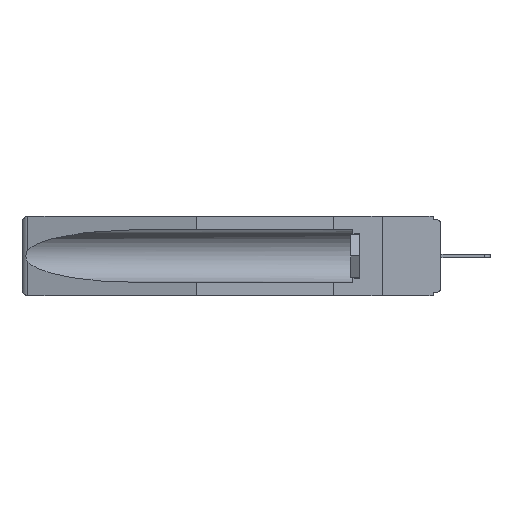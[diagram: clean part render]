
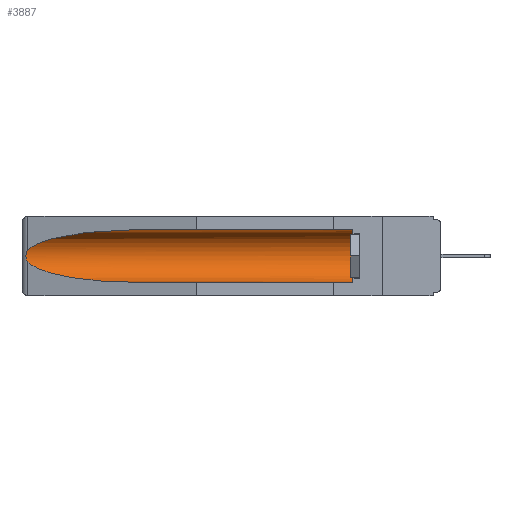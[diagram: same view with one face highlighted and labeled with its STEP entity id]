
A CAD part, left-side view. The second image highlights one B-rep face of the part: STEP entity #3887.
In plain terms, the highlighted cylindrical face has radius 2.857 mm (diameter 5.715 mm), a partial arc.
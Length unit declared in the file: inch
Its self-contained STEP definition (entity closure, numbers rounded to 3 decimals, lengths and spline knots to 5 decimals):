
#314 = ORIENTED_EDGE ( 'NONE', *, *, #5196, .T. ) ;
#578 = ORIENTED_EDGE ( 'NONE', *, *, #16388, .T. ) ;
#771 = LINE ( 'NONE', #19062, #4233 ) ;
#824 = DIRECTION ( 'NONE',  ( 0., 1., 0. ) ) ;
#1317 = CARTESIAN_POINT ( 'NONE',  ( 0.155, 0.126, -0.059 ) ) ;
#1935 = ORIENTED_EDGE ( 'NONE', *, *, #16936, .T. ) ;
#2026 = CARTESIAN_POINT ( 'NONE',  ( 0.26654, 1.53092, -0.15636 ) ) ;
#2137 = EDGE_LOOP ( 'NONE', ( #578, #15532, #16564, #17056, #314, #1935 ) ) ;
#2679 = CARTESIAN_POINT ( 'NONE',  ( 0.25451, 1.48313, -0.09465 ) ) ;
#2711 = CIRCLE ( 'NONE', #20135, 0.1125 ) ;
#3272 = CARTESIAN_POINT ( 'NONE',  ( 0.155, 1.07973, -0.284 ) ) ;
#3365 = CARTESIAN_POINT ( 'NONE',  ( 0.2673, 1.5327, -0.16383 ) ) ;
#3508 = EDGE_CURVE ( 'NONE', #16926, #14531, #14075, .T. ) ;
#3515 = CARTESIAN_POINT ( 'NONE',  ( 0.26537, 1.52718, -0.14972 ) ) ;
#3887 = ADVANCED_FACE ( 'NONE', ( #14743 ), #18563, .F. ) ;
#4233 = VECTOR ( 'NONE', #7584, 39.37008 ) ;
#4523 = CARTESIAN_POINT ( 'NONE',  ( 0.26597, 1.52961, -0.15275 ) ) ;
#4742 = LINE ( 'NONE', #20721, #17485 ) ;
#4766 = CARTESIAN_POINT ( 'NONE',  ( 0.155, 0.126, -0.284 ) ) ;
#4902 = CARTESIAN_POINT ( 'NONE',  ( 0.26537, 1.52718, -0.19328 ) ) ;
#5196 = EDGE_CURVE ( 'NONE', #18263, #14725, #2711, .T. ) ;
#5709 =( BOUNDED_CURVE ( )  B_SPLINE_CURVE ( 3, ( #4902, #6613, #18158, #8332 ),
 .UNSPECIFIED., .F., .T. ) 
 B_SPLINE_CURVE_WITH_KNOTS ( ( 4, 4 ),
 ( 0.1948, 1.5708 ),
 .UNSPECIFIED. ) 
 CURVE ( )  GEOMETRIC_REPRESENTATION_ITEM ( )  RATIONAL_B_SPLINE_CURVE ( ( 1., 0.848, 0.848, 1. ) ) 
 REPRESENTATION_ITEM ( '' )  );
#6241 =( BOUNDED_CURVE ( )  B_SPLINE_CURVE ( 3, ( #11069, #12725, #2679, #14359 ),
 .UNSPECIFIED., .F., .T. ) 
 B_SPLINE_CURVE_WITH_KNOTS ( ( 4, 4 ),
 ( 4.71239, 6.08839 ),
 .UNSPECIFIED. ) 
 CURVE ( )  GEOMETRIC_REPRESENTATION_ITEM ( )  RATIONAL_B_SPLINE_CURVE ( ( 1., 0.848, 0.848, 1. ) ) 
 REPRESENTATION_ITEM ( '' )  );
#6613 = CARTESIAN_POINT ( 'NONE',  ( 0.25451, 1.48313, -0.24835 ) ) ;
#7584 = DIRECTION ( 'NONE',  ( 0., 1., 0. ) ) ;
#7674 = DIRECTION ( 'NONE',  ( 0., -1., 0. ) ) ;
#7695 = CARTESIAN_POINT ( 'NONE',  ( 0.155, 0.126, -0.1715 ) ) ;
#7696 = DIRECTION ( 'NONE',  ( 0., 1., 0. ) ) ;
#8154 = CARTESIAN_POINT ( 'NONE',  ( 0.26537, 1.52718, -0.19328 ) ) ;
#8237 = CARTESIAN_POINT ( 'NONE',  ( 0.26597, 1.5296, -0.19026 ) ) ;
#8256 = CARTESIAN_POINT ( 'NONE',  ( 0.26655, 1.53094, -0.18657 ) ) ;
#8332 = CARTESIAN_POINT ( 'NONE',  ( 0.155, 1.07973, -0.284 ) ) ;
#8429 = CARTESIAN_POINT ( 'NONE',  ( 0.2673, 1.53269, -0.17917 ) ) ;
#8586 = AXIS2_PLACEMENT_3D ( 'NONE', #8738, #7696, #19431 ) ;
#8663 = CARTESIAN_POINT ( 'NONE',  ( 0.2675, 1.53308, -0.17534 ) ) ;
#8708 = CARTESIAN_POINT ( 'NONE',  ( 0.2675, 1.53308, -0.16763 ) ) ;
#8738 = CARTESIAN_POINT ( 'NONE',  ( 0.155, -0.30754, -0.1715 ) ) ;
#9200 = CARTESIAN_POINT ( 'NONE',  ( 0.26537, 1.52718, -0.19328 ) ) ;
#11069 = CARTESIAN_POINT ( 'NONE',  ( 0.155, 1.07973, -0.059 ) ) ;
#12725 = CARTESIAN_POINT ( 'NONE',  ( 0.21114, 1.30732, -0.059 ) ) ;
#14075 = B_SPLINE_CURVE_WITH_KNOTS ( 'NONE', 3,
 ( #3515, #4523, #2026, #3365, #8708, #8663, #8429, #8256, #8237, #8154 ),
 .UNSPECIFIED., .F., .F.,
 ( 4, 2, 2, 2, 4 ),
 ( 0., 0.00029, 0.00058, 0.00087, 0.00117 ),
 .UNSPECIFIED. ) ;
#14359 = CARTESIAN_POINT ( 'NONE',  ( 0.26537, 1.52718, -0.14972 ) ) ;
#14531 = VERTEX_POINT ( 'NONE', #9200 ) ;
#14725 = VERTEX_POINT ( 'NONE', #1317 ) ;
#14743 = FACE_OUTER_BOUND ( 'NONE', #2137, .T. ) ;
#15108 = DIRECTION ( 'NONE',  ( 0., 0., 1. ) ) ;
#15532 = ORIENTED_EDGE ( 'NONE', *, *, #3508, .T. ) ;
#15844 = CARTESIAN_POINT ( 'NONE',  ( 0.26537, 1.52718, -0.14972 ) ) ;
#16008 = VERTEX_POINT ( 'NONE', #3272 ) ;
#16339 = EDGE_CURVE ( 'NONE', #18263, #16008, #771, .T. ) ;
#16388 = EDGE_CURVE ( 'NONE', #18579, #16926, #6241, .T. ) ;
#16564 = ORIENTED_EDGE ( 'NONE', *, *, #20987, .T. ) ;
#16926 = VERTEX_POINT ( 'NONE', #15844 ) ;
#16936 = EDGE_CURVE ( 'NONE', #14725, #18579, #4742, .T. ) ;
#17056 = ORIENTED_EDGE ( 'NONE', *, *, #16339, .F. ) ;
#17199 = CARTESIAN_POINT ( 'NONE',  ( 0.155, 1.07973, -0.059 ) ) ;
#17485 = VECTOR ( 'NONE', #824, 39.37008 ) ;
#18158 = CARTESIAN_POINT ( 'NONE',  ( 0.21114, 1.30732, -0.284 ) ) ;
#18263 = VERTEX_POINT ( 'NONE', #4766 ) ;
#18563 = CYLINDRICAL_SURFACE ( 'NONE', #8586, 0.1125 ) ;
#18579 = VERTEX_POINT ( 'NONE', #17199 ) ;
#19062 = CARTESIAN_POINT ( 'NONE',  ( 0.155, -0.30754, -0.284 ) ) ;
#19431 = DIRECTION ( 'NONE',  ( 0., 0., 1. ) ) ;
#20135 = AXIS2_PLACEMENT_3D ( 'NONE', #7695, #7674, #15108 ) ;
#20721 = CARTESIAN_POINT ( 'NONE',  ( 0.155, -0.30754, -0.059 ) ) ;
#20987 = EDGE_CURVE ( 'NONE', #14531, #16008, #5709, .T. ) ;
